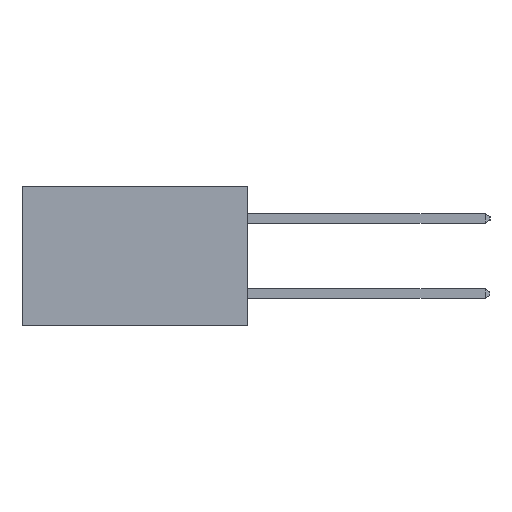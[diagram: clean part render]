
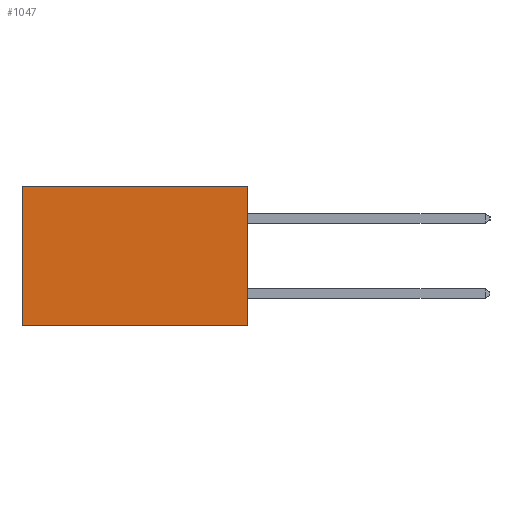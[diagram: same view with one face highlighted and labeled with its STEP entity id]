
A CAD part, left-side view. The second image highlights one B-rep face of the part: STEP entity #1047.
In plain terms, the highlighted planar face has unit normal (-1, 0, 0).
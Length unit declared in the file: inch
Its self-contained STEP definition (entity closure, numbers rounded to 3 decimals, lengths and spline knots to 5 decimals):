
#51 = ORIENTED_EDGE ( 'NONE', *, *, #19384, .F. ) ;
#534 = VERTEX_POINT ( 'NONE', #10242 ) ;
#1047 = ADVANCED_FACE ( 'NONE', ( #9588 ), #25281, .F. ) ;
#1501 = CARTESIAN_POINT ( 'NONE',  ( 0.2615, 0., 0. ) ) ;
#1936 = EDGE_LOOP ( 'NONE', ( #7117, #51, #16732, #17214 ) ) ;
#5483 = VECTOR ( 'NONE', #22337, 39.37008 ) ;
#5622 = DIRECTION ( 'NONE',  ( 0., 1., 0. ) ) ;
#6288 = CARTESIAN_POINT ( 'NONE',  ( 0.2615, 0.6, -0.37 ) ) ;
#7117 = ORIENTED_EDGE ( 'NONE', *, *, #26550, .T. ) ;
#8572 = DIRECTION ( 'NONE',  ( 0., 0., -1. ) ) ;
#9588 = FACE_OUTER_BOUND ( 'NONE', #1936, .T. ) ;
#9882 = AXIS2_PLACEMENT_3D ( 'NONE', #14320, #24489, #23120 ) ;
#10242 = CARTESIAN_POINT ( 'NONE',  ( 0.2615, 0.6, 0. ) ) ;
#10805 = LINE ( 'NONE', #25005, #16286 ) ;
#11036 = CARTESIAN_POINT ( 'NONE',  ( 0.2615, 0., 0. ) ) ;
#11314 = VECTOR ( 'NONE', #5622, 39.37008 ) ;
#12250 = DIRECTION ( 'NONE',  ( 0., 1., 0. ) ) ;
#14320 = CARTESIAN_POINT ( 'NONE',  ( 0.2615, 0., -0.37 ) ) ;
#14481 = VERTEX_POINT ( 'NONE', #19241 ) ;
#15238 = VERTEX_POINT ( 'NONE', #11036 ) ;
#16286 = VECTOR ( 'NONE', #8572, 39.37008 ) ;
#16732 = ORIENTED_EDGE ( 'NONE', *, *, #25513, .F. ) ;
#17214 = ORIENTED_EDGE ( 'NONE', *, *, #19965, .T. ) ;
#17447 = LINE ( 'NONE', #1501, #11314 ) ;
#19241 = CARTESIAN_POINT ( 'NONE',  ( 0.2615, 0., -0.37 ) ) ;
#19384 = EDGE_CURVE ( 'NONE', #14481, #23489, #21293, .T. ) ;
#19965 = EDGE_CURVE ( 'NONE', #15238, #534, #17447, .T. ) ;
#20302 = CARTESIAN_POINT ( 'NONE',  ( 0.2615, 0.6, -0.37 ) ) ;
#20660 = VECTOR ( 'NONE', #12250, 39.37008 ) ;
#21293 = LINE ( 'NONE', #22433, #20660 ) ;
#21969 = LINE ( 'NONE', #20302, #5483 ) ;
#22337 = DIRECTION ( 'NONE',  ( 0., 0., -1. ) ) ;
#22433 = CARTESIAN_POINT ( 'NONE',  ( 0.2615, 0., -0.37 ) ) ;
#23120 = DIRECTION ( 'NONE',  ( 0., 0., -1. ) ) ;
#23489 = VERTEX_POINT ( 'NONE', #6288 ) ;
#24489 = DIRECTION ( 'NONE',  ( 1., 0., 0. ) ) ;
#25005 = CARTESIAN_POINT ( 'NONE',  ( 0.2615, 0., -0.37 ) ) ;
#25281 = PLANE ( 'NONE',  #9882 ) ;
#25513 = EDGE_CURVE ( 'NONE', #15238, #14481, #10805, .T. ) ;
#26550 = EDGE_CURVE ( 'NONE', #534, #23489, #21969, .T. ) ;
